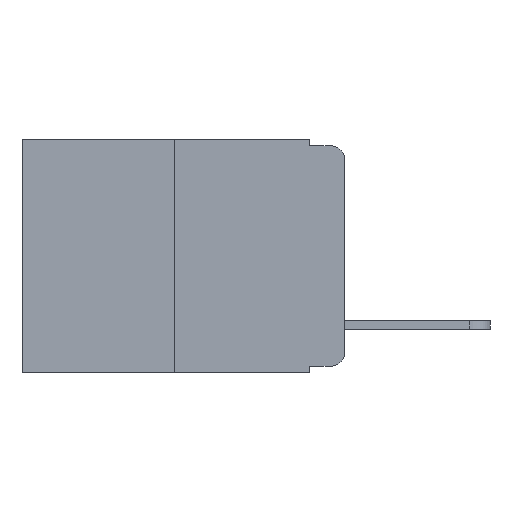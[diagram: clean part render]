
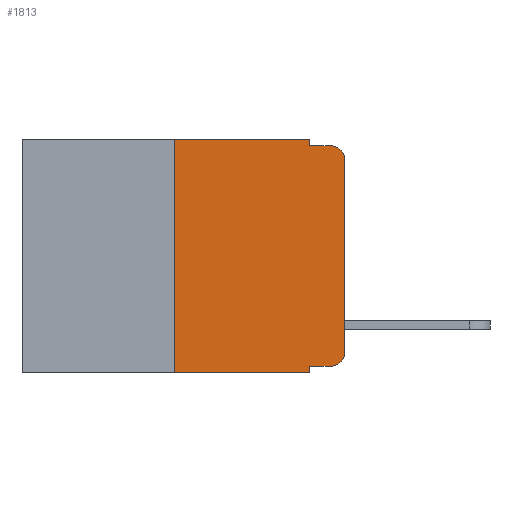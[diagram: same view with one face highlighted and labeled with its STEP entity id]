
A CAD part, left-side view. The second image highlights one B-rep face of the part: STEP entity #1813.
In plain terms, the highlighted planar face has unit normal (-1, 0, 0).
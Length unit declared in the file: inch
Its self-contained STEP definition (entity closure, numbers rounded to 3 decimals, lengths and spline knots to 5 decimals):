
#944 = CARTESIAN_POINT ( 'NONE',  ( 0., 0.02, -0.01 ) ) ;
#1322 = ORIENTED_EDGE ( 'NONE', *, *, #19984, .F. ) ;
#1502 = ORIENTED_EDGE ( 'NONE', *, *, #19267, .T. ) ;
#1503 = DIRECTION ( 'NONE',  ( 0., 0., -1. ) ) ;
#1695 = ORIENTED_EDGE ( 'NONE', *, *, #8213, .F. ) ;
#1813 = ADVANCED_FACE ( 'NONE', ( #18961 ), #16910, .F. ) ;
#2147 = VERTEX_POINT ( 'NONE', #2262 ) ;
#2262 = CARTESIAN_POINT ( 'NONE',  ( 0., 0.051, 0. ) ) ;
#2367 = VERTEX_POINT ( 'NONE', #944 ) ;
#2674 = DIRECTION ( 'NONE',  ( -1., 0., 0. ) ) ;
#2811 = CARTESIAN_POINT ( 'NONE',  ( 0., 0.473, 0. ) ) ;
#3388 = CARTESIAN_POINT ( 'NONE',  ( 0., 0.051, -0.01 ) ) ;
#3454 = CARTESIAN_POINT ( 'NONE',  ( 0., 0., -0.03 ) ) ;
#3592 = CARTESIAN_POINT ( 'NONE',  ( 0., 0., 0. ) ) ;
#3972 = LINE ( 'NONE', #3592, #21441 ) ;
#4267 = VERTEX_POINT ( 'NONE', #20702 ) ;
#4968 = DIRECTION ( 'NONE',  ( 0., -1., 0. ) ) ;
#5990 = VECTOR ( 'NONE', #21589, 39.37008 ) ;
#6053 = VECTOR ( 'NONE', #22277, 39.37008 ) ;
#6175 = VERTEX_POINT ( 'NONE', #3388 ) ;
#6508 = ORIENTED_EDGE ( 'NONE', *, *, #20718, .F. ) ;
#6583 = CIRCLE ( 'NONE', #13883, 0.02 ) ;
#6817 = CARTESIAN_POINT ( 'NONE',  ( 0., 0.473, -0.343 ) ) ;
#6828 = CARTESIAN_POINT ( 'NONE',  ( 0., 0.051, -0.333 ) ) ;
#6915 = VECTOR ( 'NONE', #8798, 39.37008 ) ;
#6920 = CARTESIAN_POINT ( 'NONE',  ( 0., 0.051, -0.01 ) ) ;
#8213 = EDGE_CURVE ( 'NONE', #6175, #2367, #11892, .T. ) ;
#8250 = DIRECTION ( 'NONE',  ( 0., 0., -1. ) ) ;
#8371 = LINE ( 'NONE', #6817, #22574 ) ;
#8622 = VERTEX_POINT ( 'NONE', #9976 ) ;
#8742 = DIRECTION ( 'NONE',  ( 0., 0., 1. ) ) ;
#8769 = VECTOR ( 'NONE', #4968, 39.37008 ) ;
#8798 = DIRECTION ( 'NONE',  ( 0., -1., 0. ) ) ;
#8910 = ORIENTED_EDGE ( 'NONE', *, *, #10715, .T. ) ;
#9369 = ORIENTED_EDGE ( 'NONE', *, *, #18199, .F. ) ;
#9976 = CARTESIAN_POINT ( 'NONE',  ( 0., 0., -0.313 ) ) ;
#10228 = LINE ( 'NONE', #19297, #6915 ) ;
#10380 = DIRECTION ( 'NONE',  ( 0., -1., 0. ) ) ;
#10424 = AXIS2_PLACEMENT_3D ( 'NONE', #2811, #16753, #8250 ) ;
#10715 = EDGE_CURVE ( 'NONE', #21428, #2367, #6583, .T. ) ;
#10716 = CARTESIAN_POINT ( 'NONE',  ( 0., 0.25, -0.343 ) ) ;
#10736 = CARTESIAN_POINT ( 'NONE',  ( 0., 0.02, -0.03 ) ) ;
#11071 = VECTOR ( 'NONE', #10380, 39.37008 ) ;
#11223 = VERTEX_POINT ( 'NONE', #10716 ) ;
#11892 = LINE ( 'NONE', #6920, #11071 ) ;
#12081 = LINE ( 'NONE', #13515, #8769 ) ;
#12086 = LINE ( 'NONE', #17019, #6053 ) ;
#12108 = VERTEX_POINT ( 'NONE', #13329 ) ;
#12588 = CIRCLE ( 'NONE', #21782, 0.02 ) ;
#12630 = DIRECTION ( 'NONE',  ( -1., 0., 0. ) ) ;
#12882 = EDGE_CURVE ( 'NONE', #11223, #12108, #8371, .T. ) ;
#13329 = CARTESIAN_POINT ( 'NONE',  ( 0., 0.051, -0.343 ) ) ;
#13515 = CARTESIAN_POINT ( 'NONE',  ( 0., 0.473, 0. ) ) ;
#13532 = CARTESIAN_POINT ( 'NONE',  ( 0., 0.051, 0. ) ) ;
#13883 = AXIS2_PLACEMENT_3D ( 'NONE', #10736, #12630, #15999 ) ;
#14032 = EDGE_CURVE ( 'NONE', #8622, #21428, #3972, .T. ) ;
#14469 = VERTEX_POINT ( 'NONE', #20225 ) ;
#14614 = VERTEX_POINT ( 'NONE', #6828 ) ;
#14777 = CARTESIAN_POINT ( 'NONE',  ( 0., 0.02, -0.313 ) ) ;
#15387 = DIRECTION ( 'NONE',  ( 0., -1., 0. ) ) ;
#15587 = LINE ( 'NONE', #21811, #5990 ) ;
#15999 = DIRECTION ( 'NONE',  ( 0., 0., -1. ) ) ;
#16541 = ORIENTED_EDGE ( 'NONE', *, *, #18667, .F. ) ;
#16753 = DIRECTION ( 'NONE',  ( 1., 0., 0. ) ) ;
#16844 = DIRECTION ( 'NONE',  ( 0., 0., -1. ) ) ;
#16910 = PLANE ( 'NONE',  #10424 ) ;
#17019 = CARTESIAN_POINT ( 'NONE',  ( 0., 0.25, 0. ) ) ;
#17030 = EDGE_CURVE ( 'NONE', #14614, #14469, #10228, .T. ) ;
#17184 = LINE ( 'NONE', #13532, #22365 ) ;
#17268 = EDGE_LOOP ( 'NONE', ( #21000, #8910, #1695, #1322, #9369, #16541, #21189, #6508, #18500, #1502 ) ) ;
#18199 = EDGE_CURVE ( 'NONE', #4267, #2147, #12081, .T. ) ;
#18500 = ORIENTED_EDGE ( 'NONE', *, *, #17030, .T. ) ;
#18667 = EDGE_CURVE ( 'NONE', #11223, #4267, #12086, .T. ) ;
#18961 = FACE_OUTER_BOUND ( 'NONE', #17268, .T. ) ;
#19267 = EDGE_CURVE ( 'NONE', #14469, #8622, #12588, .T. ) ;
#19297 = CARTESIAN_POINT ( 'NONE',  ( 0., 0.051, -0.333 ) ) ;
#19984 = EDGE_CURVE ( 'NONE', #2147, #6175, #15587, .T. ) ;
#20225 = CARTESIAN_POINT ( 'NONE',  ( 0., 0.02, -0.333 ) ) ;
#20702 = CARTESIAN_POINT ( 'NONE',  ( 0., 0.25, 0. ) ) ;
#20718 = EDGE_CURVE ( 'NONE', #14614, #12108, #17184, .T. ) ;
#21000 = ORIENTED_EDGE ( 'NONE', *, *, #14032, .T. ) ;
#21189 = ORIENTED_EDGE ( 'NONE', *, *, #12882, .T. ) ;
#21428 = VERTEX_POINT ( 'NONE', #3454 ) ;
#21441 = VECTOR ( 'NONE', #8742, 39.37008 ) ;
#21589 = DIRECTION ( 'NONE',  ( 0., 0., -1. ) ) ;
#21782 = AXIS2_PLACEMENT_3D ( 'NONE', #14777, #2674, #16844 ) ;
#21811 = CARTESIAN_POINT ( 'NONE',  ( 0., 0.051, 0. ) ) ;
#22277 = DIRECTION ( 'NONE',  ( 0., 0., 1. ) ) ;
#22365 = VECTOR ( 'NONE', #1503, 39.37008 ) ;
#22574 = VECTOR ( 'NONE', #15387, 39.37008 ) ;
